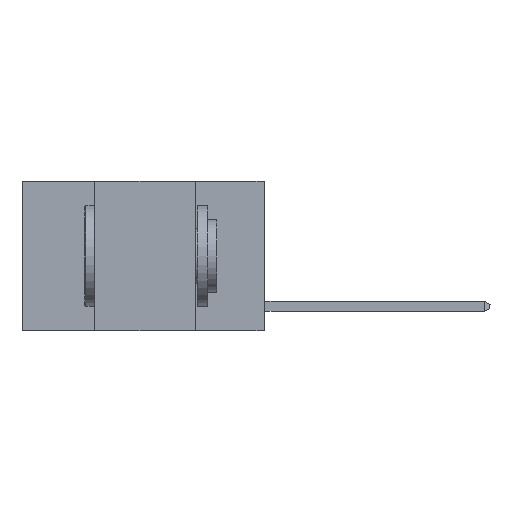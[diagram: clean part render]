
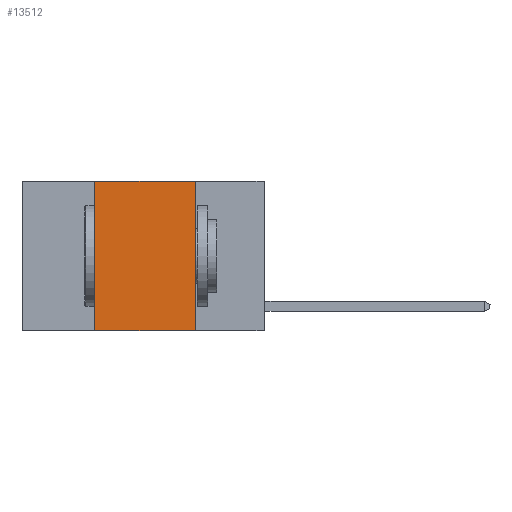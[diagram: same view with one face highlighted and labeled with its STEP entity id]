
A CAD part, left-side view. The second image highlights one B-rep face of the part: STEP entity #13512.
In plain terms, the highlighted planar face has unit normal (-1, 0, 0).
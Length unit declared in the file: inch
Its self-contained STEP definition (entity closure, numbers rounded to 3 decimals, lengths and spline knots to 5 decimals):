
#260 = AXIS2_PLACEMENT_3D ( 'NONE', #2013, #5152, #4173 ) ;
#413 = CARTESIAN_POINT ( 'NONE',  ( 0., 0.17, -0.37 ) ) ;
#484 = CARTESIAN_POINT ( 'NONE',  ( 0., 0.42, 0. ) ) ;
#1585 = CARTESIAN_POINT ( 'NONE',  ( 0., 0.6, -0.37 ) ) ;
#2013 = CARTESIAN_POINT ( 'NONE',  ( 0., 0.6, 0. ) ) ;
#2527 = LINE ( 'NONE', #18196, #12982 ) ;
#3573 = LINE ( 'NONE', #484, #18217 ) ;
#3682 = CARTESIAN_POINT ( 'NONE',  ( 0., 0.42, -0.37 ) ) ;
#4020 = EDGE_CURVE ( 'NONE', #9224, #4540, #15777, .T. ) ;
#4173 = DIRECTION ( 'NONE',  ( 0., 0., -1. ) ) ;
#4540 = VERTEX_POINT ( 'NONE', #413 ) ;
#4711 = VECTOR ( 'NONE', #12108, 39.37008 ) ;
#5152 = DIRECTION ( 'NONE',  ( 1., 0., 0. ) ) ;
#5486 = VERTEX_POINT ( 'NONE', #20410 ) ;
#6029 = ORIENTED_EDGE ( 'NONE', *, *, #4020, .T. ) ;
#6084 = VECTOR ( 'NONE', #14023, 39.37008 ) ;
#6184 = EDGE_CURVE ( 'NONE', #5486, #16494, #2527, .T. ) ;
#7158 = LINE ( 'NONE', #15207, #4711 ) ;
#8341 = CARTESIAN_POINT ( 'NONE',  ( 0., 0.17, 0. ) ) ;
#8941 = EDGE_LOOP ( 'NONE', ( #19963, #17591, #18398, #6029 ) ) ;
#8942 = FACE_OUTER_BOUND ( 'NONE', #8941, .T. ) ;
#9224 = VERTEX_POINT ( 'NONE', #3682 ) ;
#11057 = DIRECTION ( 'NONE',  ( 0., 0., 1. ) ) ;
#12108 = DIRECTION ( 'NONE',  ( 0., 0., -1. ) ) ;
#12982 = VECTOR ( 'NONE', #15172, 39.37008 ) ;
#13512 = ADVANCED_FACE ( 'NONE', ( #8942 ), #18387, .F. ) ;
#14023 = DIRECTION ( 'NONE',  ( 0., -1., 0. ) ) ;
#15172 = DIRECTION ( 'NONE',  ( 0., -1., 0. ) ) ;
#15207 = CARTESIAN_POINT ( 'NONE',  ( 0., 0.17, 0. ) ) ;
#15777 = LINE ( 'NONE', #1585, #6084 ) ;
#15826 = EDGE_CURVE ( 'NONE', #9224, #5486, #3573, .T. ) ;
#16494 = VERTEX_POINT ( 'NONE', #8341 ) ;
#17591 = ORIENTED_EDGE ( 'NONE', *, *, #6184, .F. ) ;
#18196 = CARTESIAN_POINT ( 'NONE',  ( 0., 0.6, 0. ) ) ;
#18217 = VECTOR ( 'NONE', #11057, 39.37008 ) ;
#18387 = PLANE ( 'NONE',  #260 ) ;
#18398 = ORIENTED_EDGE ( 'NONE', *, *, #15826, .F. ) ;
#18463 = EDGE_CURVE ( 'NONE', #16494, #4540, #7158, .T. ) ;
#19963 = ORIENTED_EDGE ( 'NONE', *, *, #18463, .F. ) ;
#20410 = CARTESIAN_POINT ( 'NONE',  ( 0., 0.42, 0. ) ) ;
